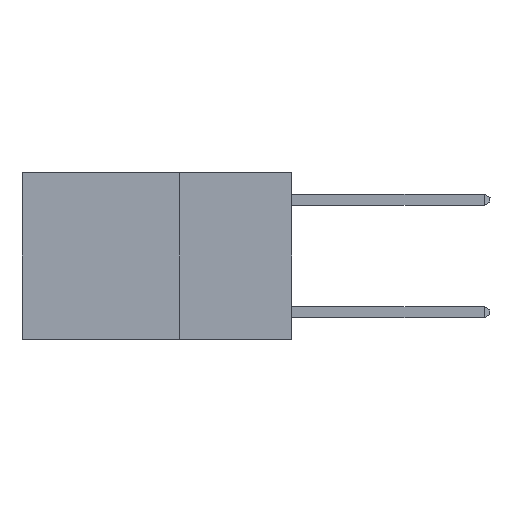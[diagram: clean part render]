
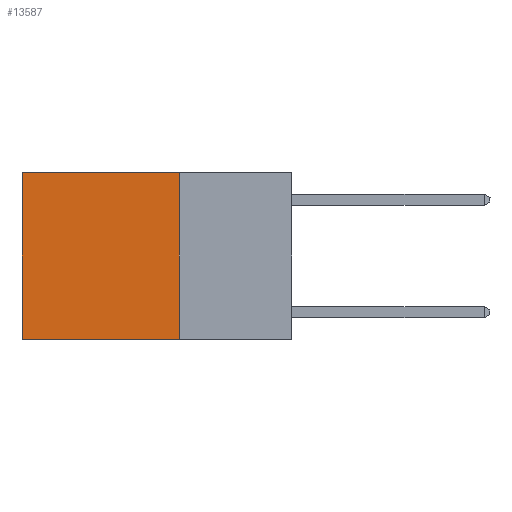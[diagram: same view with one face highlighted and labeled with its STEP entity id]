
A CAD part, left-side view. The second image highlights one B-rep face of the part: STEP entity #13587.
In plain terms, the highlighted planar face has unit normal (-1, 0, 0).
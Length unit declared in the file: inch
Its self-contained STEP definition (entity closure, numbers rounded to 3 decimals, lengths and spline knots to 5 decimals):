
#625 = DIRECTION ( 'NONE',  ( 0., 0., -1. ) ) ;
#1069 = DIRECTION ( 'NONE',  ( 0., 0., -1. ) ) ;
#1696 = VECTOR ( 'NONE', #625, 39.37008 ) ;
#2476 = VERTEX_POINT ( 'NONE', #8397 ) ;
#3135 = EDGE_LOOP ( 'NONE', ( #16210, #17374, #4198, #6589 ) ) ;
#3497 = LINE ( 'NONE', #23277, #1696 ) ;
#3686 = DIRECTION ( 'NONE',  ( 0., 1., 0. ) ) ;
#4198 = ORIENTED_EDGE ( 'NONE', *, *, #17262, .F. ) ;
#4301 = LINE ( 'NONE', #23814, #4890 ) ;
#4890 = VECTOR ( 'NONE', #1069, 39.37008 ) ;
#5550 = VERTEX_POINT ( 'NONE', #20499 ) ;
#6469 = CARTESIAN_POINT ( 'NONE',  ( 0.2625, 0.25, -0.37 ) ) ;
#6589 = ORIENTED_EDGE ( 'NONE', *, *, #12425, .T. ) ;
#6679 = CARTESIAN_POINT ( 'NONE',  ( 0.2625, 0.25, 0. ) ) ;
#7946 = VECTOR ( 'NONE', #23077, 39.37008 ) ;
#8397 = CARTESIAN_POINT ( 'NONE',  ( 0.2625, 0.6, -0.37 ) ) ;
#10465 = DIRECTION ( 'NONE',  ( 0., 0., -1. ) ) ;
#11072 = CARTESIAN_POINT ( 'NONE',  ( 0.2625, 0.25, 0. ) ) ;
#11654 = CARTESIAN_POINT ( 'NONE',  ( 0.2625, 0.25, -0.37 ) ) ;
#12081 = LINE ( 'NONE', #11072, #20930 ) ;
#12425 = EDGE_CURVE ( 'NONE', #5550, #22820, #12081, .T. ) ;
#12578 = EDGE_CURVE ( 'NONE', #14759, #2476, #23020, .T. ) ;
#13587 = ADVANCED_FACE ( 'NONE', ( #21157 ), #19864, .F. ) ;
#14759 = VERTEX_POINT ( 'NONE', #6469 ) ;
#16210 = ORIENTED_EDGE ( 'NONE', *, *, #18685, .T. ) ;
#17262 = EDGE_CURVE ( 'NONE', #5550, #14759, #3497, .T. ) ;
#17374 = ORIENTED_EDGE ( 'NONE', *, *, #12578, .F. ) ;
#17564 = CARTESIAN_POINT ( 'NONE',  ( 0.2625, 0.6, 0. ) ) ;
#18685 = EDGE_CURVE ( 'NONE', #22820, #2476, #4301, .T. ) ;
#19864 = PLANE ( 'NONE',  #22448 ) ;
#20499 = CARTESIAN_POINT ( 'NONE',  ( 0.2625, 0.25, 0. ) ) ;
#20930 = VECTOR ( 'NONE', #3686, 39.37008 ) ;
#21157 = FACE_OUTER_BOUND ( 'NONE', #3135, .T. ) ;
#21781 = DIRECTION ( 'NONE',  ( 1., 0., 0. ) ) ;
#22448 = AXIS2_PLACEMENT_3D ( 'NONE', #6679, #21781, #10465 ) ;
#22820 = VERTEX_POINT ( 'NONE', #17564 ) ;
#23020 = LINE ( 'NONE', #11654, #7946 ) ;
#23077 = DIRECTION ( 'NONE',  ( 0., 1., 0. ) ) ;
#23277 = CARTESIAN_POINT ( 'NONE',  ( 0.2625, 0.25, 0. ) ) ;
#23814 = CARTESIAN_POINT ( 'NONE',  ( 0.2625, 0.6, 0. ) ) ;
